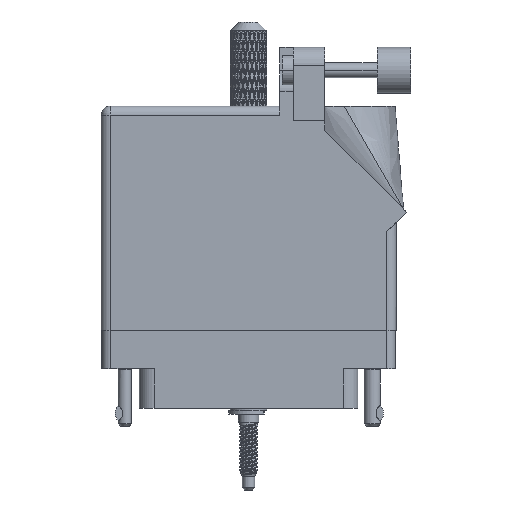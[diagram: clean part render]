
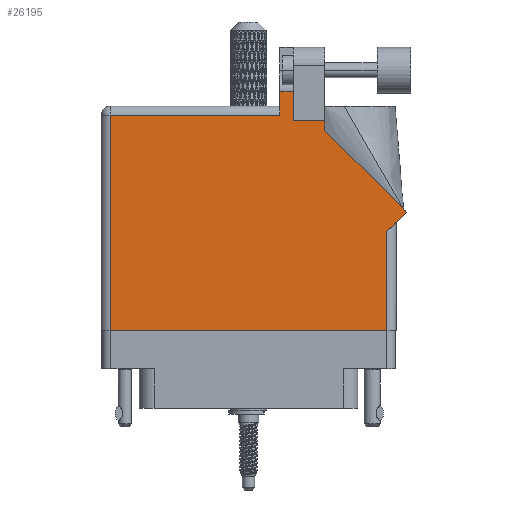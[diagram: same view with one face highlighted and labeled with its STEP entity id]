
A CAD part, front view. The second image highlights one B-rep face of the part: STEP entity #26195.
In plain terms, the highlighted face is planar.
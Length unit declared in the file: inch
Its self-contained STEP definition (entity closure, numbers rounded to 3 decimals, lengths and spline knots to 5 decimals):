
#889 = EDGE_CURVE ( 'NONE', #59399, #111296, #76917, .T. ) ;
#1803 = CARTESIAN_POINT ( 'NONE',  ( 0., 1.468, 0. ) ) ;
#3153 = VECTOR ( 'NONE', #95731, 39.37008 ) ;
#4756 = EDGE_CURVE ( 'NONE', #47396, #72563, #101375, .T. ) ;
#6754 = CARTESIAN_POINT ( 'NONE',  ( 1.217, 1.53, 0. ) ) ;
#7144 = PLANE ( 'NONE',  #89057 ) ;
#7445 = EDGE_CURVE ( 'NONE', #111296, #30147, #85944, .T. ) ;
#10217 = LINE ( 'NONE', #81298, #50894 ) ;
#10403 = EDGE_CURVE ( 'NONE', #38841, #18048, #78481, .T. ) ;
#13257 = ORIENTED_EDGE ( 'NONE', *, *, #7445, .T. ) ;
#14501 = DIRECTION ( 'NONE',  ( -1., 0., 0. ) ) ;
#14628 = CARTESIAN_POINT ( 'NONE',  ( 0.062, 0., 0. ) ) ;
#17971 = ORIENTED_EDGE ( 'NONE', *, *, #28240, .T. ) ;
#18048 = VERTEX_POINT ( 'NONE', #36129 ) ;
#18873 = DIRECTION ( 'NONE',  ( 0., 1., 0. ) ) ;
#19414 = VECTOR ( 'NONE', #27305, 39.37008 ) ;
#19674 = LINE ( 'NONE', #114081, #94599 ) ;
#19793 = ORIENTED_EDGE ( 'NONE', *, *, #4756, .T. ) ;
#20998 = CARTESIAN_POINT ( 'NONE',  ( 2.08071, 0.80771, 0. ) ) ;
#21601 = CARTESIAN_POINT ( 'NONE',  ( 1.948, 0.675, 0. ) ) ;
#21672 = CARTESIAN_POINT ( 'NONE',  ( 1.311, 1.6315, 0. ) ) ;
#25039 = CARTESIAN_POINT ( 'NONE',  ( 0., 1.53, 0. ) ) ;
#25621 = CARTESIAN_POINT ( 'NONE',  ( 1.217, 1.468, 0. ) ) ;
#25664 = DIRECTION ( 'NONE',  ( -1., 0., 0. ) ) ;
#26195 = ADVANCED_FACE ( 'NONE', ( #49959 ), #7144, .F. ) ;
#27305 = DIRECTION ( 'NONE',  ( 0., -1., 0. ) ) ;
#28240 = EDGE_CURVE ( 'NONE', #33791, #62192, #97294, .T. ) ;
#29694 = VECTOR ( 'NONE', #53160, 39.37008 ) ;
#30147 = VERTEX_POINT ( 'NONE', #25621 ) ;
#30658 = VECTOR ( 'NONE', #49386, 39.37008 ) ;
#32395 = CARTESIAN_POINT ( 'NONE',  ( 1.64177, 1.6315, 0. ) ) ;
#33396 = DIRECTION ( 'NONE',  ( 0.707, 0.707, 0. ) ) ;
#33559 = VERTEX_POINT ( 'NONE', #94840 ) ;
#33686 = CARTESIAN_POINT ( 'NONE',  ( 1.524, 1.36442, 0. ) ) ;
#33791 = VERTEX_POINT ( 'NONE', #72807 ) ;
#36129 = CARTESIAN_POINT ( 'NONE',  ( 2.08071, 0.80771, 0. ) ) ;
#37845 = VERTEX_POINT ( 'NONE', #103176 ) ;
#38841 = VERTEX_POINT ( 'NONE', #21601 ) ;
#41711 = VECTOR ( 'NONE', #33396, 39.37008 ) ;
#43933 = CARTESIAN_POINT ( 'NONE',  ( 1.948, 0.737, 0. ) ) ;
#47396 = VERTEX_POINT ( 'NONE', #14628 ) ;
#49386 = DIRECTION ( 'NONE',  ( 1., 0., 0. ) ) ;
#49642 = DIRECTION ( 'NONE',  ( -1., 0., 0. ) ) ;
#49959 = FACE_OUTER_BOUND ( 'NONE', #70451, .T. ) ;
#50894 = VECTOR ( 'NONE', #18873, 39.37008 ) ;
#51636 = DIRECTION ( 'NONE',  ( 0., 1., 0. ) ) ;
#53160 = DIRECTION ( 'NONE',  ( 0., 1., 0. ) ) ;
#54582 = LINE ( 'NONE', #20998, #113104 ) ;
#59399 = VERTEX_POINT ( 'NONE', #21672 ) ;
#62192 = VERTEX_POINT ( 'NONE', #96440 ) ;
#63123 = LINE ( 'NONE', #1803, #70711 ) ;
#64821 = DIRECTION ( 'NONE',  ( -1., 0., 0. ) ) ;
#65269 = VECTOR ( 'NONE', #51636, 39.37008 ) ;
#65477 = ORIENTED_EDGE ( 'NONE', *, *, #78105, .T. ) ;
#69370 = CARTESIAN_POINT ( 'NONE',  ( 1.217, 1.6315, 0. ) ) ;
#70287 = EDGE_CURVE ( 'NONE', #62192, #37845, #19674, .T. ) ;
#70451 = EDGE_LOOP ( 'NONE', ( #65477, #80085, #13257, #109845, #100874, #19793, #82798, #74858, #103636, #17971, #81277 ) ) ;
#70711 = VECTOR ( 'NONE', #64821, 39.37008 ) ;
#72563 = VERTEX_POINT ( 'NONE', #102305 ) ;
#72807 = CARTESIAN_POINT ( 'NONE',  ( 1.524, 1.36442, 0. ) ) ;
#74858 = ORIENTED_EDGE ( 'NONE', *, *, #10403, .T. ) ;
#76917 = LINE ( 'NONE', #32395, #97749 ) ;
#78105 = EDGE_CURVE ( 'NONE', #37845, #59399, #10217, .T. ) ;
#78366 = EDGE_CURVE ( 'NONE', #33559, #47396, #97257, .T. ) ;
#78481 = LINE ( 'NONE', #112595, #41711 ) ;
#80085 = ORIENTED_EDGE ( 'NONE', *, *, #889, .T. ) ;
#81277 = ORIENTED_EDGE ( 'NONE', *, *, #70287, .T. ) ;
#81298 = CARTESIAN_POINT ( 'NONE',  ( 1.311, 1.43, 0. ) ) ;
#82296 = DIRECTION ( 'NONE',  ( -0.707, 0.707, 0. ) ) ;
#82798 = ORIENTED_EDGE ( 'NONE', *, *, #104319, .T. ) ;
#84878 = DIRECTION ( 'NONE',  ( 0., 0., -1. ) ) ;
#85944 = LINE ( 'NONE', #6754, #3153 ) ;
#88023 = CARTESIAN_POINT ( 'NONE',  ( 0.062, 0., 0. ) ) ;
#89057 = AXIS2_PLACEMENT_3D ( 'NONE', #25039, #84878, #49642 ) ;
#94599 = VECTOR ( 'NONE', #25664, 39.37008 ) ;
#94840 = CARTESIAN_POINT ( 'NONE',  ( 0.062, 1.468, 0. ) ) ;
#95731 = DIRECTION ( 'NONE',  ( 0., -1., 0. ) ) ;
#96440 = CARTESIAN_POINT ( 'NONE',  ( 1.524, 1.43, 0. ) ) ;
#97257 = LINE ( 'NONE', #88023, #19414 ) ;
#97294 = LINE ( 'NONE', #33686, #65269 ) ;
#97749 = VECTOR ( 'NONE', #14501, 39.37008 ) ;
#98757 = LINE ( 'NONE', #43933, #29694 ) ;
#100874 = ORIENTED_EDGE ( 'NONE', *, *, #78366, .T. ) ;
#101375 = LINE ( 'NONE', #110582, #30658 ) ;
#102305 = CARTESIAN_POINT ( 'NONE',  ( 1.948, 0., 0. ) ) ;
#103176 = CARTESIAN_POINT ( 'NONE',  ( 1.311, 1.43, 0. ) ) ;
#103636 = ORIENTED_EDGE ( 'NONE', *, *, #108785, .T. ) ;
#104319 = EDGE_CURVE ( 'NONE', #72563, #38841, #98757, .T. ) ;
#108785 = EDGE_CURVE ( 'NONE', #18048, #33791, #54582, .T. ) ;
#109845 = ORIENTED_EDGE ( 'NONE', *, *, #110169, .T. ) ;
#110169 = EDGE_CURVE ( 'NONE', #30147, #33559, #63123, .T. ) ;
#110582 = CARTESIAN_POINT ( 'NONE',  ( 0., 0., 0. ) ) ;
#111296 = VERTEX_POINT ( 'NONE', #69370 ) ;
#112595 = CARTESIAN_POINT ( 'NONE',  ( 2.01, 0.737, 0. ) ) ;
#113104 = VECTOR ( 'NONE', #82296, 39.37008 ) ;
#114081 = CARTESIAN_POINT ( 'NONE',  ( 1.524, 1.43, 0. ) ) ;
